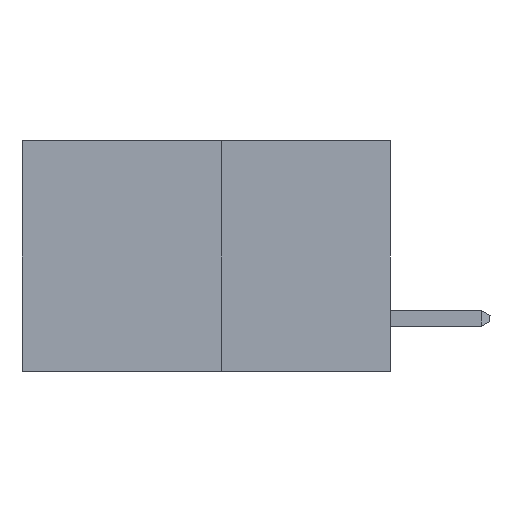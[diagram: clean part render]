
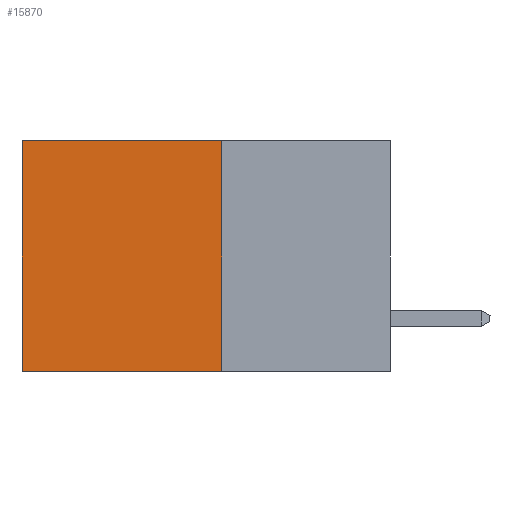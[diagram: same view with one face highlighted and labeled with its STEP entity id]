
A CAD part, left-side view. The second image highlights one B-rep face of the part: STEP entity #15870.
In plain terms, the highlighted planar face has unit normal (-1, 0, 0).
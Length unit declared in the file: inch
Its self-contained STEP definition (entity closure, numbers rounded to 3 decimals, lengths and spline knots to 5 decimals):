
#593 = EDGE_CURVE ( 'NONE', #17346, #17565, #9104, .T. ) ;
#1086 = VECTOR ( 'NONE', #6546, 39.37008 ) ;
#1340 = VERTEX_POINT ( 'NONE', #5525 ) ;
#2012 = AXIS2_PLACEMENT_3D ( 'NONE', #14841, #6481, #16269 ) ;
#2172 = ORIENTED_EDGE ( 'NONE', *, *, #10797, .F. ) ;
#2284 = EDGE_CURVE ( 'NONE', #17672, #1340, #12967, .T. ) ;
#2956 = CARTESIAN_POINT ( 'NONE',  ( 0.277, 0.27, 0. ) ) ;
#3828 = ORIENTED_EDGE ( 'NONE', *, *, #593, .T. ) ;
#4416 = DIRECTION ( 'NONE',  ( 0., 0., -1. ) ) ;
#4839 = VECTOR ( 'NONE', #4416, 39.37008 ) ;
#5525 = CARTESIAN_POINT ( 'NONE',  ( 0.277, 0.59, -0.37 ) ) ;
#5885 = CARTESIAN_POINT ( 'NONE',  ( 0.277, 0.59, -0.37 ) ) ;
#6187 = DIRECTION ( 'NONE',  ( 0., 1., 0. ) ) ;
#6481 = DIRECTION ( 'NONE',  ( 1., 0., 0. ) ) ;
#6546 = DIRECTION ( 'NONE',  ( 0., 0., -1. ) ) ;
#6744 = CARTESIAN_POINT ( 'NONE',  ( 0.277, 0.27, -0.37 ) ) ;
#8087 = CARTESIAN_POINT ( 'NONE',  ( 0.277, 0.27, -0.37 ) ) ;
#8093 = ORIENTED_EDGE ( 'NONE', *, *, #14870, .T. ) ;
#8173 = ORIENTED_EDGE ( 'NONE', *, *, #2284, .F. ) ;
#8408 = VECTOR ( 'NONE', #6187, 39.37008 ) ;
#8601 = LINE ( 'NONE', #5885, #4839 ) ;
#9104 = LINE ( 'NONE', #13141, #15652 ) ;
#9344 = CARTESIAN_POINT ( 'NONE',  ( 0.277, 0.27, -0.37 ) ) ;
#10797 = EDGE_CURVE ( 'NONE', #17346, #17672, #16185, .T. ) ;
#12025 = PLANE ( 'NONE',  #2012 ) ;
#12967 = LINE ( 'NONE', #6744, #8408 ) ;
#13141 = CARTESIAN_POINT ( 'NONE',  ( 0.277, 0.27, 0. ) ) ;
#13535 = EDGE_LOOP ( 'NONE', ( #8093, #8173, #2172, #3828 ) ) ;
#14771 = CARTESIAN_POINT ( 'NONE',  ( 0.277, 0.59, 0. ) ) ;
#14841 = CARTESIAN_POINT ( 'NONE',  ( 0.277, 0.27, -0.37 ) ) ;
#14870 = EDGE_CURVE ( 'NONE', #17565, #1340, #8601, .T. ) ;
#15494 = FACE_OUTER_BOUND ( 'NONE', #13535, .T. ) ;
#15652 = VECTOR ( 'NONE', #17285, 39.37008 ) ;
#15870 = ADVANCED_FACE ( 'NONE', ( #15494 ), #12025, .F. ) ;
#16185 = LINE ( 'NONE', #9344, #1086 ) ;
#16269 = DIRECTION ( 'NONE',  ( 0., 0., -1. ) ) ;
#17285 = DIRECTION ( 'NONE',  ( 0., 1., 0. ) ) ;
#17346 = VERTEX_POINT ( 'NONE', #2956 ) ;
#17565 = VERTEX_POINT ( 'NONE', #14771 ) ;
#17672 = VERTEX_POINT ( 'NONE', #8087 ) ;
